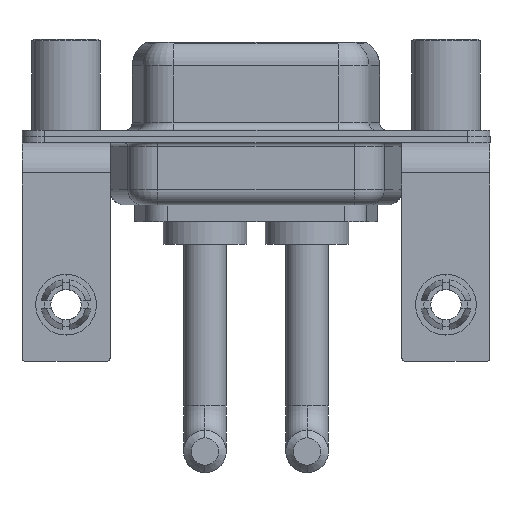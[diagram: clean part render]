
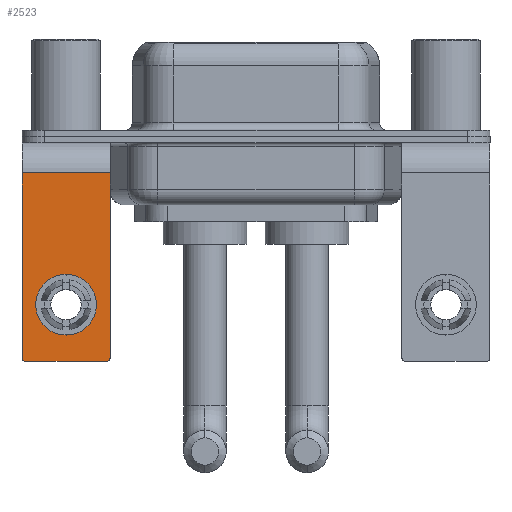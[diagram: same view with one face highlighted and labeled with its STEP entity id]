
A CAD part, front view. The second image highlights one B-rep face of the part: STEP entity #2523.
In plain terms, the highlighted planar face has unit normal (0, -1, 0).
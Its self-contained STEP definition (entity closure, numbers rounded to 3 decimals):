
#370 = EDGE_LOOP ( 'NONE', ( #9027, #14150 ) ) ;
#887 = LINE ( 'NONE', #14170, #2790 ) ;
#1187 = CARTESIAN_POINT ( 'NONE',  ( 2.9, -6.25, -14.55 ) ) ;
#1203 = EDGE_CURVE ( 'NONE', #8774, #9895, #14746, .T. ) ;
#1267 = DIRECTION ( 'NONE',  ( 0., -1., 0. ) ) ;
#1346 = DIRECTION ( 'NONE',  ( 0., 0., 1. ) ) ;
#1393 = EDGE_CURVE ( 'NONE', #11131, #8774, #8385, .T. ) ;
#1792 = CARTESIAN_POINT ( 'NONE',  ( -2.65, -6.25, -14.55 ) ) ;
#1859 = AXIS2_PLACEMENT_3D ( 'NONE', #8731, #1267, #1346 ) ;
#1958 = DIRECTION ( 'NONE',  ( -1., 0., 0. ) ) ;
#2214 = EDGE_CURVE ( 'NONE', #14120, #11131, #6741, .T. ) ;
#2293 = CARTESIAN_POINT ( 'NONE',  ( 2.9, -6.25, -2.4 ) ) ;
#2523 = ADVANCED_FACE ( 'NONE', ( #14107, #11475 ), #5501, .F. ) ;
#2790 = VECTOR ( 'NONE', #5652, 1000. ) ;
#2935 = CIRCLE ( 'NONE', #4209, 2. ) ;
#3271 = DIRECTION ( 'NONE',  ( 0., 0., 1. ) ) ;
#4055 = DIRECTION ( 'NONE',  ( 0., 1., 0. ) ) ;
#4094 = VECTOR ( 'NONE', #1958, 1000. ) ;
#4209 = AXIS2_PLACEMENT_3D ( 'NONE', #12112, #4055, #6527 ) ;
#4786 = VERTEX_POINT ( 'NONE', #5299 ) ;
#4851 = DIRECTION ( 'NONE',  ( 0., 0., 1. ) ) ;
#4908 = CIRCLE ( 'NONE', #15313, 2. ) ;
#5207 = DIRECTION ( 'NONE',  ( 0., 0., 1. ) ) ;
#5299 = CARTESIAN_POINT ( 'NONE',  ( 0., -6.25, -13.07 ) ) ;
#5501 = PLANE ( 'NONE',  #14769 ) ;
#5652 = DIRECTION ( 'NONE',  ( -1., 0., 0. ) ) ;
#6115 = DIRECTION ( 'NONE',  ( 0., 1., 0. ) ) ;
#6144 = EDGE_CURVE ( 'NONE', #8899, #9895, #887, .T. ) ;
#6527 = DIRECTION ( 'NONE',  ( 0., 0., 1. ) ) ;
#6618 = CARTESIAN_POINT ( 'NONE',  ( 0., -6.25, -9.07 ) ) ;
#6741 = LINE ( 'NONE', #12869, #4094 ) ;
#7340 = ORIENTED_EDGE ( 'NONE', *, *, #10148, .F. ) ;
#8385 = LINE ( 'NONE', #13105, #10434 ) ;
#8564 = LINE ( 'NONE', #2293, #11087 ) ;
#8577 = CARTESIAN_POINT ( 'NONE',  ( 0., -6.25, -11.07 ) ) ;
#8670 = CARTESIAN_POINT ( 'NONE',  ( -2.9, -6.25, -14.55 ) ) ;
#8731 = CARTESIAN_POINT ( 'NONE',  ( 2.65, -6.25, -14.55 ) ) ;
#8774 = VERTEX_POINT ( 'NONE', #8670 ) ;
#8864 = EDGE_CURVE ( 'NONE', #11354, #4786, #2935, .T. ) ;
#8899 = VERTEX_POINT ( 'NONE', #13855 ) ;
#9027 = ORIENTED_EDGE ( 'NONE', *, *, #15159, .T. ) ;
#9042 = ORIENTED_EDGE ( 'NONE', *, *, #15135, .T. ) ;
#9160 = DIRECTION ( 'NONE',  ( 0., 1., 0. ) ) ;
#9895 = VERTEX_POINT ( 'NONE', #12719 ) ;
#10065 = DIRECTION ( 'NONE',  ( 0., -1., 0. ) ) ;
#10148 = EDGE_CURVE ( 'NONE', #14120, #11809, #8564, .T. ) ;
#10434 = VECTOR ( 'NONE', #10702, 1000. ) ;
#10598 = CARTESIAN_POINT ( 'NONE',  ( 2.9, -6.25, -2.4 ) ) ;
#10702 = DIRECTION ( 'NONE',  ( 0., 0., -1. ) ) ;
#10936 = AXIS2_PLACEMENT_3D ( 'NONE', #1792, #10065, #5207 ) ;
#11087 = VECTOR ( 'NONE', #12156, 1000. ) ;
#11131 = VERTEX_POINT ( 'NONE', #13088 ) ;
#11354 = VERTEX_POINT ( 'NONE', #6618 ) ;
#11475 = FACE_OUTER_BOUND ( 'NONE', #11758, .T. ) ;
#11581 = ORIENTED_EDGE ( 'NONE', *, *, #1393, .T. ) ;
#11589 = ORIENTED_EDGE ( 'NONE', *, *, #1203, .T. ) ;
#11758 = EDGE_LOOP ( 'NONE', ( #11581, #11589, #13505, #9042, #7340, #13651 ) ) ;
#11809 = VERTEX_POINT ( 'NONE', #1187 ) ;
#12112 = CARTESIAN_POINT ( 'NONE',  ( 0., -6.25, -11.07 ) ) ;
#12132 = CARTESIAN_POINT ( 'NONE',  ( 2.9, -6.25, -2.4 ) ) ;
#12156 = DIRECTION ( 'NONE',  ( 0., 0., -1. ) ) ;
#12719 = CARTESIAN_POINT ( 'NONE',  ( -2.65, -6.25, -14.8 ) ) ;
#12869 = CARTESIAN_POINT ( 'NONE',  ( 2.9, -6.25, -2.4 ) ) ;
#13088 = CARTESIAN_POINT ( 'NONE',  ( -2.9, -6.25, -2.4 ) ) ;
#13105 = CARTESIAN_POINT ( 'NONE',  ( -2.9, -6.25, -2.4 ) ) ;
#13505 = ORIENTED_EDGE ( 'NONE', *, *, #6144, .F. ) ;
#13554 = CIRCLE ( 'NONE', #1859, 0.25 ) ;
#13651 = ORIENTED_EDGE ( 'NONE', *, *, #2214, .T. ) ;
#13855 = CARTESIAN_POINT ( 'NONE',  ( 2.65, -6.25, -14.8 ) ) ;
#14107 = FACE_BOUND ( 'NONE', #370, .T. ) ;
#14120 = VERTEX_POINT ( 'NONE', #12132 ) ;
#14150 = ORIENTED_EDGE ( 'NONE', *, *, #8864, .T. ) ;
#14170 = CARTESIAN_POINT ( 'NONE',  ( 2.9, -6.25, -14.8 ) ) ;
#14746 = CIRCLE ( 'NONE', #10936, 0.25 ) ;
#14769 = AXIS2_PLACEMENT_3D ( 'NONE', #10598, #9160, #3271 ) ;
#15135 = EDGE_CURVE ( 'NONE', #8899, #11809, #13554, .T. ) ;
#15159 = EDGE_CURVE ( 'NONE', #4786, #11354, #4908, .T. ) ;
#15313 = AXIS2_PLACEMENT_3D ( 'NONE', #8577, #6115, #4851 ) ;
